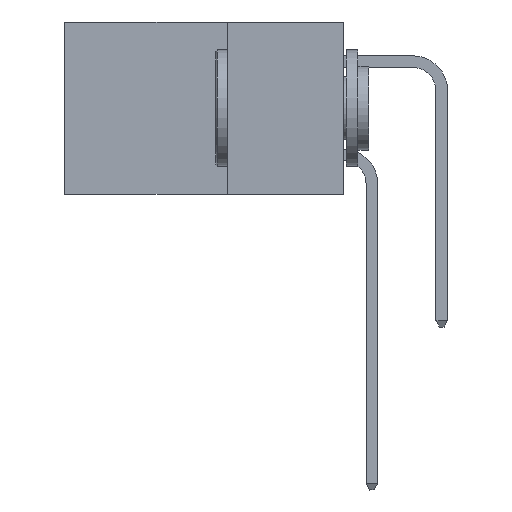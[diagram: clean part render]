
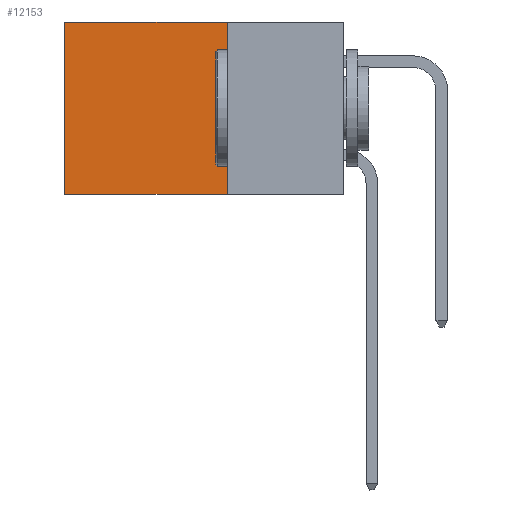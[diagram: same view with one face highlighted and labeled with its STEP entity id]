
A CAD part, left-side view. The second image highlights one B-rep face of the part: STEP entity #12153.
In plain terms, the highlighted planar face has unit normal (-1, 0, 0).
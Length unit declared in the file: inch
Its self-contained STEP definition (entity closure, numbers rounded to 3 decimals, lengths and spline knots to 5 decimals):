
#1088 = EDGE_CURVE ( 'NONE', #25279, #20825, #9448, .T. ) ;
#2303 = VECTOR ( 'NONE', #5142, 39.37008 ) ;
#2416 = ORIENTED_EDGE ( 'NONE', *, *, #2519, .F. ) ;
#2519 = EDGE_CURVE ( 'NONE', #20825, #9196, #26655, .T. ) ;
#2765 = CARTESIAN_POINT ( 'NONE',  ( 0.2615, 0.25, 0. ) ) ;
#3164 = VECTOR ( 'NONE', #12554, 39.37008 ) ;
#5142 = DIRECTION ( 'NONE',  ( 0., 1., 0. ) ) ;
#5419 = EDGE_CURVE ( 'NONE', #23365, #9196, #13520, .T. ) ;
#5547 = CARTESIAN_POINT ( 'NONE',  ( 0.2615, 0.25, -0.37 ) ) ;
#6350 = PLANE ( 'NONE',  #24400 ) ;
#9196 = VERTEX_POINT ( 'NONE', #19839 ) ;
#9448 = LINE ( 'NONE', #21089, #26733 ) ;
#10344 = EDGE_LOOP ( 'NONE', ( #24520, #2416, #11212, #15615 ) ) ;
#11027 = DIRECTION ( 'NONE',  ( 0., 0., -1. ) ) ;
#11212 = ORIENTED_EDGE ( 'NONE', *, *, #1088, .F. ) ;
#11469 = DIRECTION ( 'NONE',  ( 0., 0., -1. ) ) ;
#12153 = ADVANCED_FACE ( 'NONE', ( #17998 ), #6350, .F. ) ;
#12554 = DIRECTION ( 'NONE',  ( 0., 1., 0. ) ) ;
#13154 = CARTESIAN_POINT ( 'NONE',  ( 0.2615, 0.25, -0.37 ) ) ;
#13239 = EDGE_CURVE ( 'NONE', #25279, #23365, #14719, .T. ) ;
#13520 = LINE ( 'NONE', #21766, #18186 ) ;
#14719 = LINE ( 'NONE', #2765, #2303 ) ;
#15615 = ORIENTED_EDGE ( 'NONE', *, *, #13239, .T. ) ;
#16650 = CARTESIAN_POINT ( 'NONE',  ( 0.2615, 0.6, 0. ) ) ;
#17998 = FACE_OUTER_BOUND ( 'NONE', #10344, .T. ) ;
#18186 = VECTOR ( 'NONE', #19544, 39.37008 ) ;
#19544 = DIRECTION ( 'NONE',  ( 0., 0., -1. ) ) ;
#19839 = CARTESIAN_POINT ( 'NONE',  ( 0.2615, 0.6, -0.37 ) ) ;
#20825 = VERTEX_POINT ( 'NONE', #5547 ) ;
#21089 = CARTESIAN_POINT ( 'NONE',  ( 0.2615, 0.25, -0.37 ) ) ;
#21766 = CARTESIAN_POINT ( 'NONE',  ( 0.2615, 0.6, -0.37 ) ) ;
#22321 = CARTESIAN_POINT ( 'NONE',  ( 0.2615, 0.25, -0.37 ) ) ;
#23365 = VERTEX_POINT ( 'NONE', #16650 ) ;
#24400 = AXIS2_PLACEMENT_3D ( 'NONE', #22321, #24532, #11027 ) ;
#24520 = ORIENTED_EDGE ( 'NONE', *, *, #5419, .T. ) ;
#24532 = DIRECTION ( 'NONE',  ( 1., 0., 0. ) ) ;
#25279 = VERTEX_POINT ( 'NONE', #25483 ) ;
#25483 = CARTESIAN_POINT ( 'NONE',  ( 0.2615, 0.25, 0. ) ) ;
#26655 = LINE ( 'NONE', #13154, #3164 ) ;
#26733 = VECTOR ( 'NONE', #11469, 39.37008 ) ;
